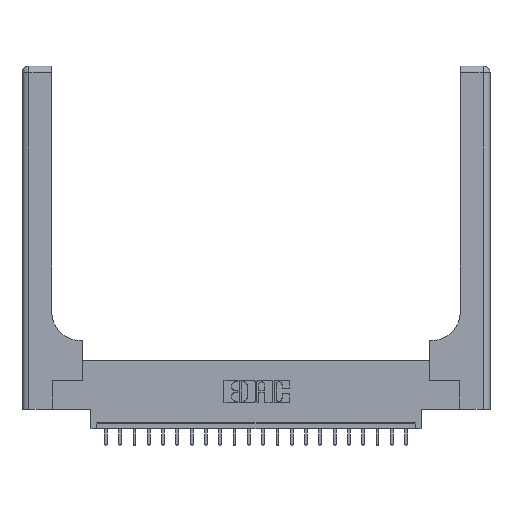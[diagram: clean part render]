
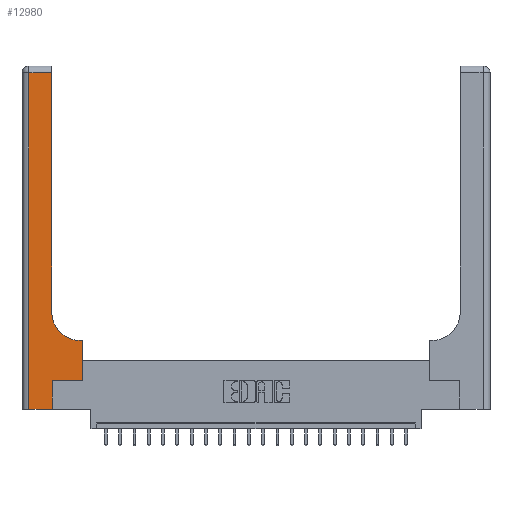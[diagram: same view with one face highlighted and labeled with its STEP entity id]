
A CAD part, top view. The second image highlights one B-rep face of the part: STEP entity #12980.
In plain terms, the highlighted planar face has unit normal (0, 0, 1).
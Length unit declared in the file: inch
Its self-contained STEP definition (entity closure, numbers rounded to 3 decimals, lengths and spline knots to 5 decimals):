
#78 = DIRECTION ( 'NONE',  ( 0., -1., 0. ) ) ;
#234 = CARTESIAN_POINT ( 'NONE',  ( 0.51, 0.6, 0.37 ) ) ;
#627 = LINE ( 'NONE', #6054, #12403 ) ;
#654 = CARTESIAN_POINT ( 'NONE',  ( 0.26, 0.6, 0.37 ) ) ;
#1368 = CARTESIAN_POINT ( 'NONE',  ( 0.265, 0., 0.37 ) ) ;
#1459 = DIRECTION ( 'NONE',  ( 1., 0., 0. ) ) ;
#1613 = ORIENTED_EDGE ( 'NONE', *, *, #14609, .T. ) ;
#1985 = LINE ( 'NONE', #6806, #13220 ) ;
#2014 = VECTOR ( 'NONE', #4126, 39.37008 ) ;
#2362 = CIRCLE ( 'NONE', #5718, 0.25 ) ;
#2550 = CARTESIAN_POINT ( 'NONE',  ( 0.265, 0.25, 0.37 ) ) ;
#2904 = VERTEX_POINT ( 'NONE', #21061 ) ;
#2964 = EDGE_CURVE ( 'NONE', #2994, #7466, #627, .T. ) ;
#2994 = VERTEX_POINT ( 'NONE', #5919 ) ;
#3531 = DIRECTION ( 'NONE',  ( 0., 0., -1. ) ) ;
#3817 = CARTESIAN_POINT ( 'NONE',  ( 0., 3., 0.37 ) ) ;
#4126 = DIRECTION ( 'NONE',  ( -1., 0., 0. ) ) ;
#4837 = ORIENTED_EDGE ( 'NONE', *, *, #2964, .T. ) ;
#5133 = VERTEX_POINT ( 'NONE', #12983 ) ;
#5718 = AXIS2_PLACEMENT_3D ( 'NONE', #19116, #10845, #5889 ) ;
#5837 = CARTESIAN_POINT ( 'NONE',  ( 0.528, 0.25, 0.37 ) ) ;
#5867 = DIRECTION ( 'NONE',  ( 0., 1., 0. ) ) ;
#5889 = DIRECTION ( 'NONE',  ( 1., 0., 0. ) ) ;
#5919 = CARTESIAN_POINT ( 'NONE',  ( 0.26, 0.85, 0.37 ) ) ;
#6054 = CARTESIAN_POINT ( 'NONE',  ( 0.26, 3., 0.37 ) ) ;
#6433 = DIRECTION ( 'NONE',  ( 0., 1., 0. ) ) ;
#6621 = CARTESIAN_POINT ( 'NONE',  ( 0.06, 0., 0.37 ) ) ;
#6709 = AXIS2_PLACEMENT_3D ( 'NONE', #3817, #3531, #13267 ) ;
#6806 = CARTESIAN_POINT ( 'NONE',  ( 0.06, 3., 0.37 ) ) ;
#7015 = VECTOR ( 'NONE', #5867, 39.37008 ) ;
#7391 = VECTOR ( 'NONE', #1459, 39.37008 ) ;
#7447 = LINE ( 'NONE', #654, #11651 ) ;
#7466 = VERTEX_POINT ( 'NONE', #21147 ) ;
#7767 = DIRECTION ( 'NONE',  ( 1., 0., 0. ) ) ;
#8328 = EDGE_CURVE ( 'NONE', #19573, #2904, #17946, .T. ) ;
#9156 = CARTESIAN_POINT ( 'NONE',  ( 0.265, 0., 0.37 ) ) ;
#9402 = CARTESIAN_POINT ( 'NONE',  ( 0.265, 0.25, 0.37 ) ) ;
#9425 = VECTOR ( 'NONE', #7767, 39.37008 ) ;
#9800 = CARTESIAN_POINT ( 'NONE',  ( 0., 0., 0.37 ) ) ;
#10845 = DIRECTION ( 'NONE',  ( 0., 0., -1. ) ) ;
#11413 = CARTESIAN_POINT ( 'NONE',  ( 0.528, 0.25, 0.37 ) ) ;
#11464 = EDGE_CURVE ( 'NONE', #20584, #2994, #2362, .T. ) ;
#11595 = EDGE_CURVE ( 'NONE', #14729, #19573, #15953, .T. ) ;
#11651 = VECTOR ( 'NONE', #15868, 39.37008 ) ;
#12403 = VECTOR ( 'NONE', #17470, 39.37008 ) ;
#12980 = ADVANCED_FACE ( 'NONE', ( #18257 ), #15399, .F. ) ;
#12983 = CARTESIAN_POINT ( 'NONE',  ( 0.06, 2.94, 0.37 ) ) ;
#13101 = ORIENTED_EDGE ( 'NONE', *, *, #11595, .T. ) ;
#13220 = VECTOR ( 'NONE', #78, 39.37008 ) ;
#13259 = LINE ( 'NONE', #14287, #2014 ) ;
#13267 = DIRECTION ( 'NONE',  ( -1., 0., 0. ) ) ;
#13494 = VECTOR ( 'NONE', #6433, 39.37008 ) ;
#14287 = CARTESIAN_POINT ( 'NONE',  ( 0., 2.94, 0.37 ) ) ;
#14296 = EDGE_LOOP ( 'NONE', ( #4837, #16518, #16995, #20283, #20229, #13101, #17994, #1613, #20506 ) ) ;
#14374 = EDGE_CURVE ( 'NONE', #5133, #17626, #1985, .T. ) ;
#14609 = EDGE_CURVE ( 'NONE', #2904, #20584, #7447, .T. ) ;
#14729 = VERTEX_POINT ( 'NONE', #2550 ) ;
#15399 = PLANE ( 'NONE',  #6709 ) ;
#15868 = DIRECTION ( 'NONE',  ( -1., 0., 0. ) ) ;
#15953 = LINE ( 'NONE', #9402, #9425 ) ;
#15978 = VERTEX_POINT ( 'NONE', #1368 ) ;
#16518 = ORIENTED_EDGE ( 'NONE', *, *, #18124, .T. ) ;
#16941 = EDGE_CURVE ( 'NONE', #15978, #14729, #21432, .T. ) ;
#16995 = ORIENTED_EDGE ( 'NONE', *, *, #14374, .T. ) ;
#17470 = DIRECTION ( 'NONE',  ( 0., 1., 0. ) ) ;
#17626 = VERTEX_POINT ( 'NONE', #6621 ) ;
#17946 = LINE ( 'NONE', #11413, #13494 ) ;
#17994 = ORIENTED_EDGE ( 'NONE', *, *, #8328, .T. ) ;
#18124 = EDGE_CURVE ( 'NONE', #7466, #5133, #13259, .T. ) ;
#18257 = FACE_OUTER_BOUND ( 'NONE', #14296, .T. ) ;
#19116 = CARTESIAN_POINT ( 'NONE',  ( 0.51, 0.85, 0.37 ) ) ;
#19573 = VERTEX_POINT ( 'NONE', #5837 ) ;
#19703 = LINE ( 'NONE', #9800, #7391 ) ;
#20229 = ORIENTED_EDGE ( 'NONE', *, *, #16941, .T. ) ;
#20283 = ORIENTED_EDGE ( 'NONE', *, *, #21042, .T. ) ;
#20506 = ORIENTED_EDGE ( 'NONE', *, *, #11464, .T. ) ;
#20584 = VERTEX_POINT ( 'NONE', #234 ) ;
#21042 = EDGE_CURVE ( 'NONE', #17626, #15978, #19703, .T. ) ;
#21061 = CARTESIAN_POINT ( 'NONE',  ( 0.528, 0.6, 0.37 ) ) ;
#21147 = CARTESIAN_POINT ( 'NONE',  ( 0.26, 2.94, 0.37 ) ) ;
#21432 = LINE ( 'NONE', #9156, #7015 ) ;
